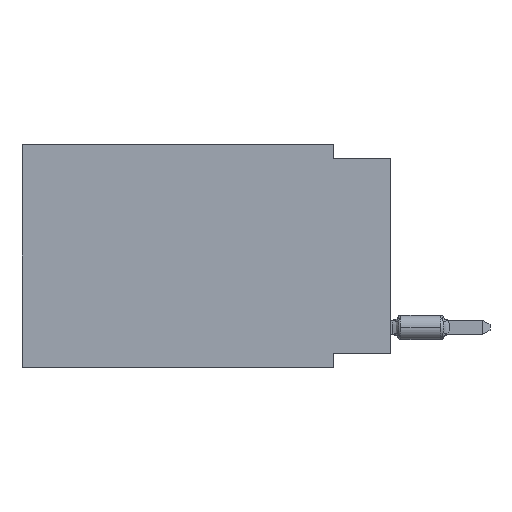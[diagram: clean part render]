
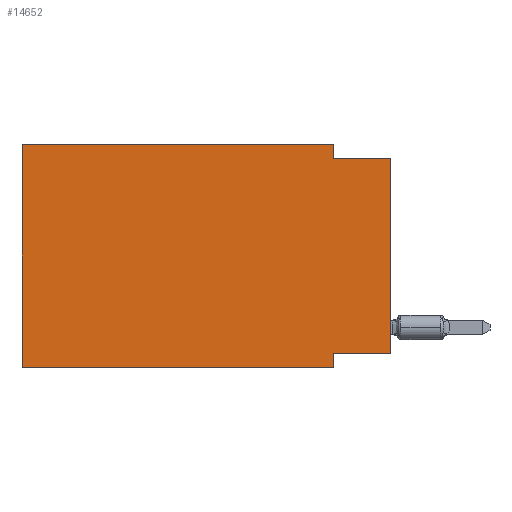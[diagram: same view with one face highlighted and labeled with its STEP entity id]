
A CAD part, left-side view. The second image highlights one B-rep face of the part: STEP entity #14652.
In plain terms, the highlighted planar face has unit normal (-1, 0, 0).
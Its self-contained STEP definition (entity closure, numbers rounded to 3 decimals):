
#185 = LINE ( 'NONE', #2883, #16517 ) ;
#295 = EDGE_CURVE ( 'NONE', #1291, #3323, #9369, .T. ) ;
#548 = EDGE_CURVE ( 'NONE', #3323, #14126, #14325, .T. ) ;
#883 = VECTOR ( 'NONE', #8398, 1000. ) ;
#1084 = CARTESIAN_POINT ( 'NONE',  ( 0., 0., -9.271 ) ) ;
#1169 = DIRECTION ( 'NONE',  ( 0., 0., -1. ) ) ;
#1291 = VERTEX_POINT ( 'NONE', #18071 ) ;
#1314 = CARTESIAN_POINT ( 'NONE',  ( 0., 16.383, -9.906 ) ) ;
#1606 = CARTESIAN_POINT ( 'NONE',  ( 0., 0., -9.271 ) ) ;
#1806 = FACE_OUTER_BOUND ( 'NONE', #8798, .T. ) ;
#1840 = CARTESIAN_POINT ( 'NONE',  ( 0., 0., 0. ) ) ;
#2138 = EDGE_CURVE ( 'NONE', #14969, #13561, #15863, .T. ) ;
#2883 = CARTESIAN_POINT ( 'NONE',  ( 0., 2.54, -9.906 ) ) ;
#3009 = DIRECTION ( 'NONE',  ( 0., 0., -1. ) ) ;
#3323 = VERTEX_POINT ( 'NONE', #9538 ) ;
#3844 = EDGE_CURVE ( 'NONE', #10570, #13561, #11246, .T. ) ;
#4318 = VECTOR ( 'NONE', #1169, 1000. ) ;
#4629 = DIRECTION ( 'NONE',  ( 0., 0., -1. ) ) ;
#4711 = DIRECTION ( 'NONE',  ( 0., -1., 0. ) ) ;
#4833 = VECTOR ( 'NONE', #6964, 1000. ) ;
#4926 = VECTOR ( 'NONE', #13029, 1000. ) ;
#5803 = ORIENTED_EDGE ( 'NONE', *, *, #15095, .T. ) ;
#6430 = VECTOR ( 'NONE', #4711, 1000. ) ;
#6468 = LINE ( 'NONE', #1084, #15277 ) ;
#6964 = DIRECTION ( 'NONE',  ( 0., -1., 0. ) ) ;
#7291 = ORIENTED_EDGE ( 'NONE', *, *, #295, .F. ) ;
#7441 = CARTESIAN_POINT ( 'NONE',  ( 0., 16.383, 0. ) ) ;
#7750 = CARTESIAN_POINT ( 'NONE',  ( 0., 2.54, -9.906 ) ) ;
#7931 = EDGE_CURVE ( 'NONE', #14126, #10570, #13827, .T. ) ;
#8204 = VECTOR ( 'NONE', #10569, 1000. ) ;
#8350 = LINE ( 'NONE', #1314, #4833 ) ;
#8395 = ORIENTED_EDGE ( 'NONE', *, *, #8951, .F. ) ;
#8398 = DIRECTION ( 'NONE',  ( 0., -1., 0. ) ) ;
#8500 = ORIENTED_EDGE ( 'NONE', *, *, #548, .F. ) ;
#8612 = CARTESIAN_POINT ( 'NONE',  ( 0., 16.383, 0. ) ) ;
#8798 = EDGE_LOOP ( 'NONE', ( #15289, #13057, #16726, #8500, #7291, #5803, #15480, #8395 ) ) ;
#8951 = EDGE_CURVE ( 'NONE', #14969, #16379, #6468, .T. ) ;
#9226 = CARTESIAN_POINT ( 'NONE',  ( 0., 2.54, -0.635 ) ) ;
#9369 = LINE ( 'NONE', #14983, #8204 ) ;
#9538 = CARTESIAN_POINT ( 'NONE',  ( 0., 16.383, 0. ) ) ;
#10037 = PLANE ( 'NONE',  #17483 ) ;
#10569 = DIRECTION ( 'NONE',  ( 0., 0., 1. ) ) ;
#10570 = VERTEX_POINT ( 'NONE', #9226 ) ;
#10974 = DIRECTION ( 'NONE',  ( 0., 1., 0. ) ) ;
#11187 = EDGE_CURVE ( 'NONE', #16379, #17172, #185, .T. ) ;
#11246 = LINE ( 'NONE', #15485, #883 ) ;
#12802 = CARTESIAN_POINT ( 'NONE',  ( 0., 0., -0.635 ) ) ;
#13029 = DIRECTION ( 'NONE',  ( 0., 0., 1. ) ) ;
#13057 = ORIENTED_EDGE ( 'NONE', *, *, #3844, .F. ) ;
#13561 = VERTEX_POINT ( 'NONE', #12802 ) ;
#13827 = LINE ( 'NONE', #14102, #4318 ) ;
#14102 = CARTESIAN_POINT ( 'NONE',  ( 0., 2.54, 0. ) ) ;
#14126 = VERTEX_POINT ( 'NONE', #14301 ) ;
#14301 = CARTESIAN_POINT ( 'NONE',  ( 0., 2.54, 0. ) ) ;
#14325 = LINE ( 'NONE', #8612, #6430 ) ;
#14652 = ADVANCED_FACE ( 'NONE', ( #1806 ), #10037, .F. ) ;
#14969 = VERTEX_POINT ( 'NONE', #1606 ) ;
#14983 = CARTESIAN_POINT ( 'NONE',  ( 0., 16.383, 0. ) ) ;
#15095 = EDGE_CURVE ( 'NONE', #1291, #17172, #8350, .T. ) ;
#15277 = VECTOR ( 'NONE', #10974, 1000. ) ;
#15289 = ORIENTED_EDGE ( 'NONE', *, *, #2138, .T. ) ;
#15480 = ORIENTED_EDGE ( 'NONE', *, *, #11187, .F. ) ;
#15485 = CARTESIAN_POINT ( 'NONE',  ( 0., 0., -0.635 ) ) ;
#15643 = DIRECTION ( 'NONE',  ( 1., 0., 0. ) ) ;
#15863 = LINE ( 'NONE', #1840, #4926 ) ;
#15910 = CARTESIAN_POINT ( 'NONE',  ( 0., 2.54, -9.271 ) ) ;
#16379 = VERTEX_POINT ( 'NONE', #15910 ) ;
#16517 = VECTOR ( 'NONE', #4629, 1000. ) ;
#16726 = ORIENTED_EDGE ( 'NONE', *, *, #7931, .F. ) ;
#17172 = VERTEX_POINT ( 'NONE', #7750 ) ;
#17483 = AXIS2_PLACEMENT_3D ( 'NONE', #7441, #15643, #3009 ) ;
#18071 = CARTESIAN_POINT ( 'NONE',  ( 0., 16.383, -9.906 ) ) ;
